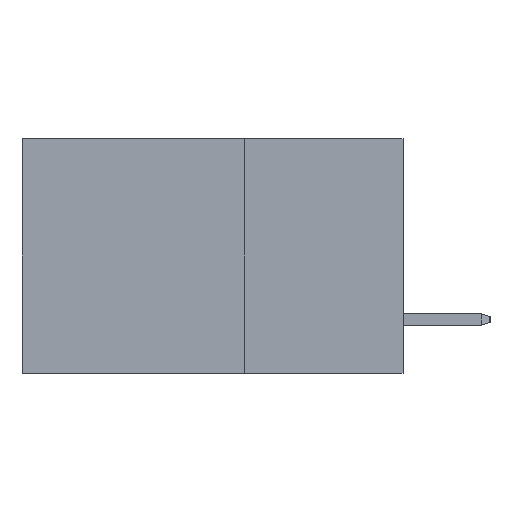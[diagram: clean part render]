
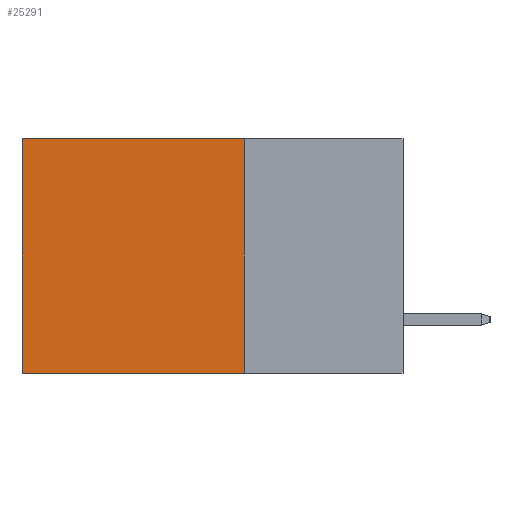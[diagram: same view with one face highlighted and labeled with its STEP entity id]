
A CAD part, left-side view. The second image highlights one B-rep face of the part: STEP entity #25291.
In plain terms, the highlighted planar face has unit normal (-1, 0, 0).
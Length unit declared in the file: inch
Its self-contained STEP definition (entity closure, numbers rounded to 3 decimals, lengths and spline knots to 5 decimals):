
#484 = PLANE ( 'NONE',  #21607 ) ;
#635 = DIRECTION ( 'NONE',  ( 0., 1., 0. ) ) ;
#1736 = ORIENTED_EDGE ( 'NONE', *, *, #11118, .T. ) ;
#2377 = LINE ( 'NONE', #13893, #3513 ) ;
#3140 = VECTOR ( 'NONE', #3633, 39.37008 ) ;
#3513 = VECTOR ( 'NONE', #13764, 39.37008 ) ;
#3633 = DIRECTION ( 'NONE',  ( 0., 0., -1. ) ) ;
#4257 = EDGE_CURVE ( 'NONE', #10398, #16553, #23104, .T. ) ;
#4757 = DIRECTION ( 'NONE',  ( 1., 0., 0. ) ) ;
#5468 = EDGE_CURVE ( 'NONE', #10398, #24792, #7769, .T. ) ;
#5660 = VERTEX_POINT ( 'NONE', #13956 ) ;
#5743 = ORIENTED_EDGE ( 'NONE', *, *, #11567, .F. ) ;
#7769 = LINE ( 'NONE', #11504, #3140 ) ;
#8650 = LINE ( 'NONE', #18451, #14661 ) ;
#9463 = EDGE_LOOP ( 'NONE', ( #1736, #5743, #19494, #21778 ) ) ;
#10398 = VERTEX_POINT ( 'NONE', #17022 ) ;
#10698 = CARTESIAN_POINT ( 'NONE',  ( 0.2875, 0.25, 0. ) ) ;
#11118 = EDGE_CURVE ( 'NONE', #16553, #5660, #2377, .T. ) ;
#11504 = CARTESIAN_POINT ( 'NONE',  ( 0.2875, 0.25, 0. ) ) ;
#11567 = EDGE_CURVE ( 'NONE', #24792, #5660, #8650, .T. ) ;
#13764 = DIRECTION ( 'NONE',  ( 0., 0., -1. ) ) ;
#13893 = CARTESIAN_POINT ( 'NONE',  ( 0.2875, 0.6, 0. ) ) ;
#13956 = CARTESIAN_POINT ( 'NONE',  ( 0.2875, 0.6, -0.37 ) ) ;
#14339 = CARTESIAN_POINT ( 'NONE',  ( 0.2875, 0.25, -0.37 ) ) ;
#14661 = VECTOR ( 'NONE', #635, 39.37008 ) ;
#16553 = VERTEX_POINT ( 'NONE', #20380 ) ;
#17022 = CARTESIAN_POINT ( 'NONE',  ( 0.2875, 0.25, 0. ) ) ;
#17047 = CARTESIAN_POINT ( 'NONE',  ( 0.2875, 0.25, 0. ) ) ;
#18451 = CARTESIAN_POINT ( 'NONE',  ( 0.2875, 0.25, -0.37 ) ) ;
#19494 = ORIENTED_EDGE ( 'NONE', *, *, #5468, .F. ) ;
#20244 = DIRECTION ( 'NONE',  ( 0., 0., -1. ) ) ;
#20380 = CARTESIAN_POINT ( 'NONE',  ( 0.2875, 0.6, 0. ) ) ;
#21181 = DIRECTION ( 'NONE',  ( 0., 1., 0. ) ) ;
#21607 = AXIS2_PLACEMENT_3D ( 'NONE', #10698, #4757, #20244 ) ;
#21778 = ORIENTED_EDGE ( 'NONE', *, *, #4257, .T. ) ;
#22432 = FACE_OUTER_BOUND ( 'NONE', #9463, .T. ) ;
#23104 = LINE ( 'NONE', #17047, #23115 ) ;
#23115 = VECTOR ( 'NONE', #21181, 39.37008 ) ;
#24792 = VERTEX_POINT ( 'NONE', #14339 ) ;
#25291 = ADVANCED_FACE ( 'NONE', ( #22432 ), #484, .F. ) ;
